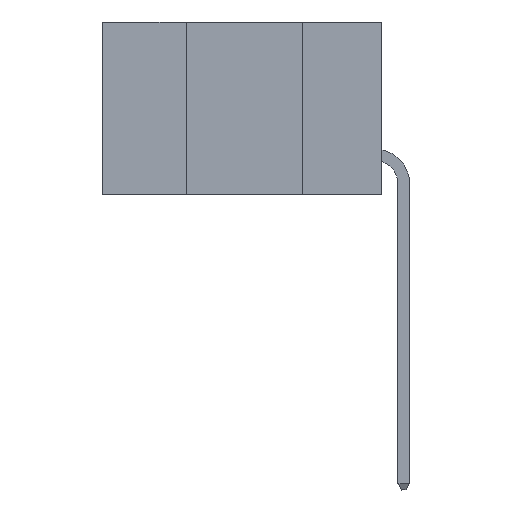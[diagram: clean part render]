
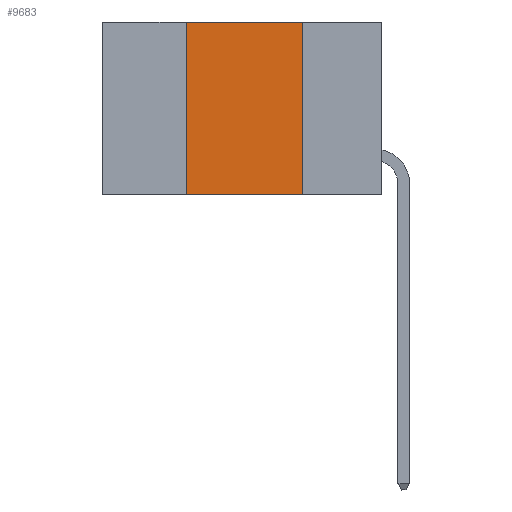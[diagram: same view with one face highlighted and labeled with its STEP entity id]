
A CAD part, left-side view. The second image highlights one B-rep face of the part: STEP entity #9683.
In plain terms, the highlighted planar face has unit normal (-1, 0, 0).
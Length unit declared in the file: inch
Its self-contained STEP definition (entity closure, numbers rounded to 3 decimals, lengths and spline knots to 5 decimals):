
#414 = LINE ( 'NONE', #33395, #14897 ) ;
#4013 = DIRECTION ( 'NONE',  ( 0., 0., 1. ) ) ;
#4354 = ORIENTED_EDGE ( 'NONE', *, *, #14075, .F. ) ;
#5931 = CARTESIAN_POINT ( 'NONE',  ( 0., 0.6, 0. ) ) ;
#6872 = ORIENTED_EDGE ( 'NONE', *, *, #8218, .F. ) ;
#8218 = EDGE_CURVE ( 'NONE', #8748, #13992, #8596, .T. ) ;
#8596 = LINE ( 'NONE', #15050, #30048 ) ;
#8748 = VERTEX_POINT ( 'NONE', #11314 ) ;
#8958 = DIRECTION ( 'NONE',  ( 0., 0., -1. ) ) ;
#9315 = DIRECTION ( 'NONE',  ( 0., -1., 0. ) ) ;
#9683 = ADVANCED_FACE ( 'NONE', ( #32058 ), #33646, .F. ) ;
#11314 = CARTESIAN_POINT ( 'NONE',  ( 0., 0.42, 0. ) ) ;
#11980 = VECTOR ( 'NONE', #4013, 39.37008 ) ;
#13962 = ORIENTED_EDGE ( 'NONE', *, *, #33253, .F. ) ;
#13992 = VERTEX_POINT ( 'NONE', #16013 ) ;
#14075 = EDGE_CURVE ( 'NONE', #32906, #8748, #15053, .T. ) ;
#14713 = DIRECTION ( 'NONE',  ( 1., 0., 0. ) ) ;
#14897 = VECTOR ( 'NONE', #8958, 39.37008 ) ;
#15050 = CARTESIAN_POINT ( 'NONE',  ( 0., 0.6, 0. ) ) ;
#15053 = LINE ( 'NONE', #20233, #11980 ) ;
#16013 = CARTESIAN_POINT ( 'NONE',  ( 0., 0.17, 0. ) ) ;
#17178 = LINE ( 'NONE', #25784, #30343 ) ;
#19905 = EDGE_LOOP ( 'NONE', ( #13962, #6872, #4354, #27573 ) ) ;
#20233 = CARTESIAN_POINT ( 'NONE',  ( 0., 0.42, 0. ) ) ;
#22389 = CARTESIAN_POINT ( 'NONE',  ( 0., 0.42, -0.37 ) ) ;
#25784 = CARTESIAN_POINT ( 'NONE',  ( 0., 0.6, -0.37 ) ) ;
#27573 = ORIENTED_EDGE ( 'NONE', *, *, #31768, .T. ) ;
#30048 = VECTOR ( 'NONE', #9315, 39.37008 ) ;
#30343 = VECTOR ( 'NONE', #33000, 39.37008 ) ;
#30601 = AXIS2_PLACEMENT_3D ( 'NONE', #5931, #14713, #32169 ) ;
#30828 = VERTEX_POINT ( 'NONE', #33803 ) ;
#31768 = EDGE_CURVE ( 'NONE', #32906, #30828, #17178, .T. ) ;
#32058 = FACE_OUTER_BOUND ( 'NONE', #19905, .T. ) ;
#32169 = DIRECTION ( 'NONE',  ( 0., 0., -1. ) ) ;
#32906 = VERTEX_POINT ( 'NONE', #22389 ) ;
#33000 = DIRECTION ( 'NONE',  ( 0., -1., 0. ) ) ;
#33253 = EDGE_CURVE ( 'NONE', #13992, #30828, #414, .T. ) ;
#33395 = CARTESIAN_POINT ( 'NONE',  ( 0., 0.17, 0. ) ) ;
#33646 = PLANE ( 'NONE',  #30601 ) ;
#33803 = CARTESIAN_POINT ( 'NONE',  ( 0., 0.17, -0.37 ) ) ;
